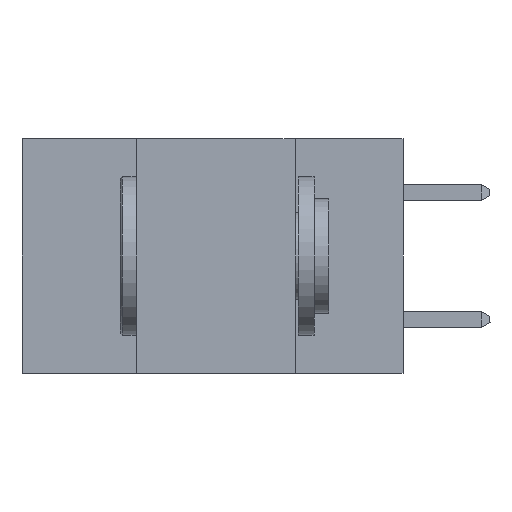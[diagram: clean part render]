
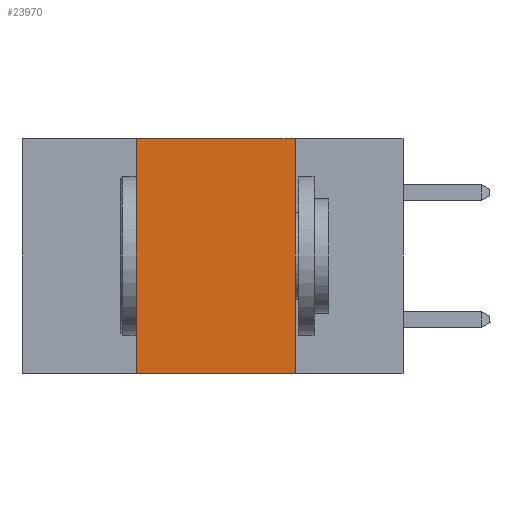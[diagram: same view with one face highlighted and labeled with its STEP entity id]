
A CAD part, left-side view. The second image highlights one B-rep face of the part: STEP entity #23970.
In plain terms, the highlighted planar face has unit normal (-1, 0, 0).
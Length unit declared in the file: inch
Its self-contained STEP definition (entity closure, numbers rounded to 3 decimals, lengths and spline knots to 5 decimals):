
#1010 = EDGE_LOOP ( 'NONE', ( #2876, #24079, #24557, #7822 ) ) ;
#1358 = CARTESIAN_POINT ( 'NONE',  ( 0., 0.17, 0. ) ) ;
#1621 = FACE_OUTER_BOUND ( 'NONE', #1010, .T. ) ;
#1627 = DIRECTION ( 'NONE',  ( 0., 0., -1. ) ) ;
#1731 = EDGE_CURVE ( 'NONE', #13271, #21690, #22084, .T. ) ;
#1926 = DIRECTION ( 'NONE',  ( 0., 0., 1. ) ) ;
#2320 = CARTESIAN_POINT ( 'NONE',  ( 0., 0.17, -0.37 ) ) ;
#2833 = VECTOR ( 'NONE', #10172, 39.37008 ) ;
#2876 = ORIENTED_EDGE ( 'NONE', *, *, #3634, .F. ) ;
#3584 = VERTEX_POINT ( 'NONE', #1358 ) ;
#3634 = EDGE_CURVE ( 'NONE', #3584, #21690, #20679, .T. ) ;
#5391 = DIRECTION ( 'NONE',  ( 0., 0., -1. ) ) ;
#6313 = CARTESIAN_POINT ( 'NONE',  ( 0., 0.42, 0. ) ) ;
#6895 = VECTOR ( 'NONE', #1926, 39.37008 ) ;
#7822 = ORIENTED_EDGE ( 'NONE', *, *, #1731, .T. ) ;
#9891 = EDGE_CURVE ( 'NONE', #13271, #20502, #12336, .T. ) ;
#10172 = DIRECTION ( 'NONE',  ( 0., -1., 0. ) ) ;
#11475 = DIRECTION ( 'NONE',  ( 1., 0., 0. ) ) ;
#11649 = AXIS2_PLACEMENT_3D ( 'NONE', #23958, #11475, #5391 ) ;
#12336 = LINE ( 'NONE', #20652, #6895 ) ;
#13271 = VERTEX_POINT ( 'NONE', #19831 ) ;
#13957 = CARTESIAN_POINT ( 'NONE',  ( 0., 0.17, 0. ) ) ;
#13972 = LINE ( 'NONE', #17282, #25855 ) ;
#14226 = EDGE_CURVE ( 'NONE', #20502, #3584, #13972, .T. ) ;
#17282 = CARTESIAN_POINT ( 'NONE',  ( 0., 0.6, 0. ) ) ;
#19100 = VECTOR ( 'NONE', #1627, 39.37008 ) ;
#19831 = CARTESIAN_POINT ( 'NONE',  ( 0., 0.42, -0.37 ) ) ;
#20502 = VERTEX_POINT ( 'NONE', #6313 ) ;
#20652 = CARTESIAN_POINT ( 'NONE',  ( 0., 0.42, 0. ) ) ;
#20679 = LINE ( 'NONE', #13957, #19100 ) ;
#21690 = VERTEX_POINT ( 'NONE', #2320 ) ;
#21769 = DIRECTION ( 'NONE',  ( 0., -1., 0. ) ) ;
#21856 = PLANE ( 'NONE',  #11649 ) ;
#22084 = LINE ( 'NONE', #22741, #2833 ) ;
#22741 = CARTESIAN_POINT ( 'NONE',  ( 0., 0.6, -0.37 ) ) ;
#23958 = CARTESIAN_POINT ( 'NONE',  ( 0., 0.6, 0. ) ) ;
#23970 = ADVANCED_FACE ( 'NONE', ( #1621 ), #21856, .F. ) ;
#24079 = ORIENTED_EDGE ( 'NONE', *, *, #14226, .F. ) ;
#24557 = ORIENTED_EDGE ( 'NONE', *, *, #9891, .F. ) ;
#25855 = VECTOR ( 'NONE', #21769, 39.37008 ) ;
